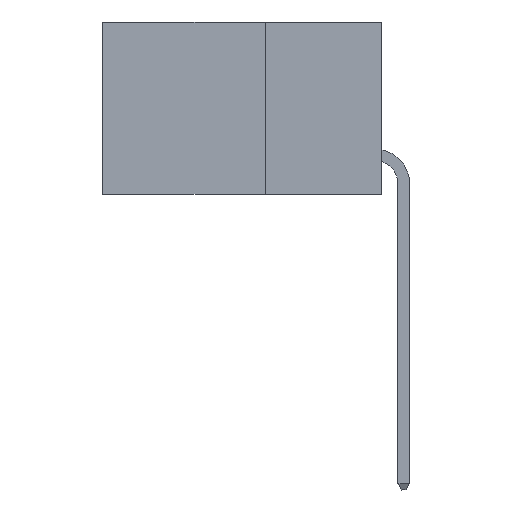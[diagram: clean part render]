
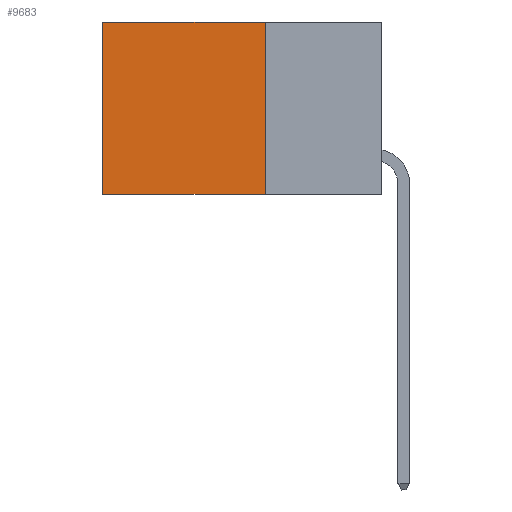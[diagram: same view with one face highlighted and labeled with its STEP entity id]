
A CAD part, left-side view. The second image highlights one B-rep face of the part: STEP entity #9683.
In plain terms, the highlighted planar face has unit normal (-1, 0, 0).
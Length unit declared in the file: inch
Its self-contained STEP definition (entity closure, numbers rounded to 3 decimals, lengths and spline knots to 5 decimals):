
#4003 = EDGE_CURVE ( 'NONE', #27263, #32881, #6682, .T. ) ;
#4950 = VECTOR ( 'NONE', #16691, 39.37008 ) ;
#6682 = LINE ( 'NONE', #29762, #38802 ) ;
#7803 = CARTESIAN_POINT ( 'NONE',  ( 0.2875, 0.6, 0. ) ) ;
#8223 = FACE_OUTER_BOUND ( 'NONE', #21588, .T. ) ;
#9683 = ADVANCED_FACE ( 'NONE', ( #8223 ), #35642, .F. ) ;
#11384 = VERTEX_POINT ( 'NONE', #37799 ) ;
#16380 = ORIENTED_EDGE ( 'NONE', *, *, #27418, .T. ) ;
#16691 = DIRECTION ( 'NONE',  ( 0., 1., 0. ) ) ;
#16973 = VECTOR ( 'NONE', #30351, 39.37008 ) ;
#16979 = DIRECTION ( 'NONE',  ( 0., 0., -1. ) ) ;
#17026 = EDGE_CURVE ( 'NONE', #27263, #20921, #32572, .T. ) ;
#17277 = AXIS2_PLACEMENT_3D ( 'NONE', #29359, #38740, #20099 ) ;
#18496 = VECTOR ( 'NONE', #16979, 39.37008 ) ;
#20099 = DIRECTION ( 'NONE',  ( 0., 0., -1. ) ) ;
#20921 = VERTEX_POINT ( 'NONE', #28382 ) ;
#21588 = EDGE_LOOP ( 'NONE', ( #16380, #40029, #30373, #37666 ) ) ;
#25454 = CARTESIAN_POINT ( 'NONE',  ( 0.2875, 0.25, 0. ) ) ;
#26259 = CARTESIAN_POINT ( 'NONE',  ( 0.2875, 0.6, 0. ) ) ;
#27263 = VERTEX_POINT ( 'NONE', #25454 ) ;
#27327 = EDGE_CURVE ( 'NONE', #20921, #11384, #38038, .T. ) ;
#27418 = EDGE_CURVE ( 'NONE', #32881, #11384, #36092, .T. ) ;
#28382 = CARTESIAN_POINT ( 'NONE',  ( 0.2875, 0.25, -0.37 ) ) ;
#29359 = CARTESIAN_POINT ( 'NONE',  ( 0.2875, 0.25, 0. ) ) ;
#29762 = CARTESIAN_POINT ( 'NONE',  ( 0.2875, 0.25, 0. ) ) ;
#30351 = DIRECTION ( 'NONE',  ( 0., 0., -1. ) ) ;
#30373 = ORIENTED_EDGE ( 'NONE', *, *, #17026, .F. ) ;
#32572 = LINE ( 'NONE', #39886, #16973 ) ;
#32881 = VERTEX_POINT ( 'NONE', #7803 ) ;
#35408 = CARTESIAN_POINT ( 'NONE',  ( 0.2875, 0.25, -0.37 ) ) ;
#35642 = PLANE ( 'NONE',  #17277 ) ;
#36055 = DIRECTION ( 'NONE',  ( 0., 1., 0. ) ) ;
#36092 = LINE ( 'NONE', #26259, #18496 ) ;
#37666 = ORIENTED_EDGE ( 'NONE', *, *, #4003, .T. ) ;
#37799 = CARTESIAN_POINT ( 'NONE',  ( 0.2875, 0.6, -0.37 ) ) ;
#38038 = LINE ( 'NONE', #35408, #4950 ) ;
#38740 = DIRECTION ( 'NONE',  ( 1., 0., 0. ) ) ;
#38802 = VECTOR ( 'NONE', #36055, 39.37008 ) ;
#39886 = CARTESIAN_POINT ( 'NONE',  ( 0.2875, 0.25, 0. ) ) ;
#40029 = ORIENTED_EDGE ( 'NONE', *, *, #27327, .F. ) ;
